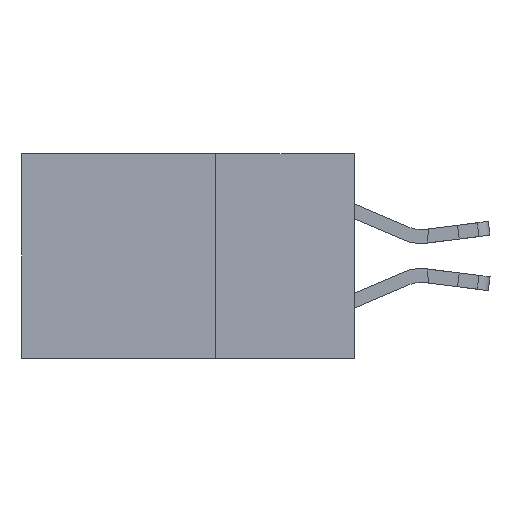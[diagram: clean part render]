
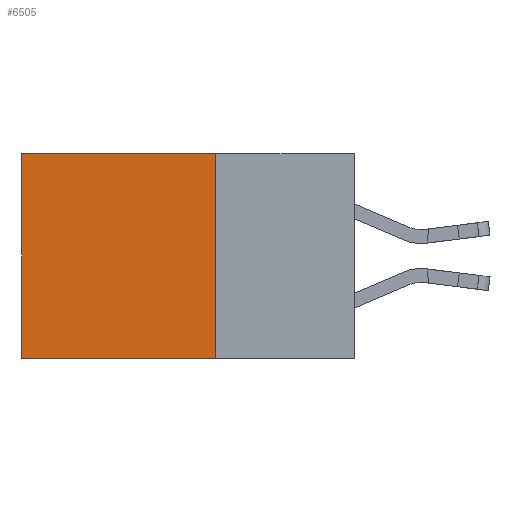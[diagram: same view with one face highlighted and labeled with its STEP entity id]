
A CAD part, left-side view. The second image highlights one B-rep face of the part: STEP entity #6505.
In plain terms, the highlighted planar face has unit normal (-1, 0, 0).
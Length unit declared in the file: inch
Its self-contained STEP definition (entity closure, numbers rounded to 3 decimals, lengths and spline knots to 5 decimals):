
#580 = VERTEX_POINT ( 'NONE', #6560 ) ;
#2341 = DIRECTION ( 'NONE',  ( 0., 0., -1. ) ) ;
#4162 = PLANE ( 'NONE',  #5360 ) ;
#4606 = VERTEX_POINT ( 'NONE', #7816 ) ;
#4936 = CARTESIAN_POINT ( 'NONE',  ( 0.298, 0.25, -0.37 ) ) ;
#5360 = AXIS2_PLACEMENT_3D ( 'NONE', #11306, #14180, #18469 ) ;
#5724 = LINE ( 'NONE', #11891, #11100 ) ;
#6505 = ADVANCED_FACE ( 'NONE', ( #15562 ), #4162, .F. ) ;
#6560 = CARTESIAN_POINT ( 'NONE',  ( 0.298, 0.6, -0.37 ) ) ;
#7816 = CARTESIAN_POINT ( 'NONE',  ( 0.298, 0.6, 0. ) ) ;
#7845 = EDGE_CURVE ( 'NONE', #4606, #580, #5724, .T. ) ;
#8000 = ORIENTED_EDGE ( 'NONE', *, *, #16376, .F. ) ;
#8843 = VERTEX_POINT ( 'NONE', #4936 ) ;
#9128 = DIRECTION ( 'NONE',  ( 0., 0., -1. ) ) ;
#9212 = DIRECTION ( 'NONE',  ( 0., 1., 0. ) ) ;
#9380 = ORIENTED_EDGE ( 'NONE', *, *, #10469, .T. ) ;
#9790 = ORIENTED_EDGE ( 'NONE', *, *, #7845, .T. ) ;
#10448 = VECTOR ( 'NONE', #2341, 39.37008 ) ;
#10469 = EDGE_CURVE ( 'NONE', #15895, #4606, #13143, .T. ) ;
#10569 = EDGE_LOOP ( 'NONE', ( #9790, #8000, #17075, #9380 ) ) ;
#10870 = EDGE_CURVE ( 'NONE', #15895, #8843, #17639, .T. ) ;
#10869 = CARTESIAN_POINT ( 'NONE',  ( 0.298, 0.25, 0. ) ) ;
#11100 = VECTOR ( 'NONE', #9128, 39.37008 ) ;
#11306 = CARTESIAN_POINT ( 'NONE',  ( 0.298, 0.25, 0. ) ) ;
#11891 = CARTESIAN_POINT ( 'NONE',  ( 0.298, 0.6, 0. ) ) ;
#11925 = CARTESIAN_POINT ( 'NONE',  ( 0.298, 0.25, 0. ) ) ;
#12093 = CARTESIAN_POINT ( 'NONE',  ( 0.298, 0.25, 0. ) ) ;
#13143 = LINE ( 'NONE', #12093, #15615 ) ;
#13470 = CARTESIAN_POINT ( 'NONE',  ( 0.298, 0.25, -0.37 ) ) ;
#13520 = DIRECTION ( 'NONE',  ( 0., 1., 0. ) ) ;
#13751 = VECTOR ( 'NONE', #9212, 39.37008 ) ;
#14180 = DIRECTION ( 'NONE',  ( 1., 0., 0. ) ) ;
#15562 = FACE_OUTER_BOUND ( 'NONE', #10569, .T. ) ;
#15615 = VECTOR ( 'NONE', #13520, 39.37008 ) ;
#15895 = VERTEX_POINT ( 'NONE', #11925 ) ;
#16376 = EDGE_CURVE ( 'NONE', #8843, #580, #17597, .T. ) ;
#17075 = ORIENTED_EDGE ( 'NONE', *, *, #10870, .F. ) ;
#17597 = LINE ( 'NONE', #13470, #13751 ) ;
#17639 = LINE ( 'NONE', #10869, #10448 ) ;
#18469 = DIRECTION ( 'NONE',  ( 0., 0., -1. ) ) ;
